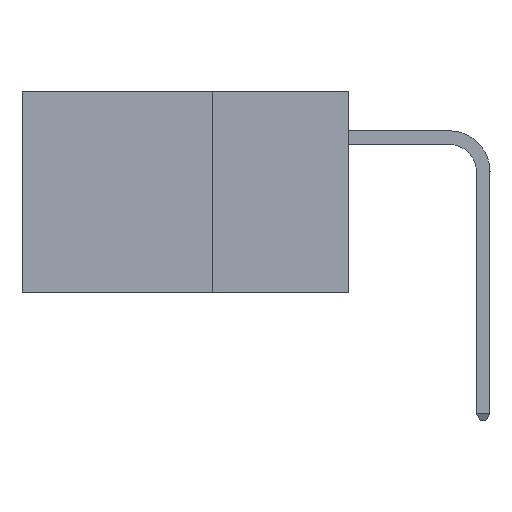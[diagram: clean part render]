
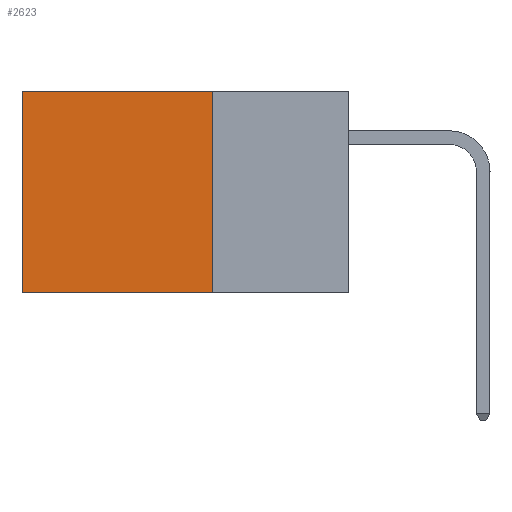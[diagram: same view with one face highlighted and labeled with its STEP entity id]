
A CAD part, left-side view. The second image highlights one B-rep face of the part: STEP entity #2623.
In plain terms, the highlighted planar face has unit normal (-1, 0, 0).
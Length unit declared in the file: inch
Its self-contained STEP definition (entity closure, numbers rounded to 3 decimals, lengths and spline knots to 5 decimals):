
#65 = PLANE ( 'NONE',  #16703 ) ;
#685 = EDGE_CURVE ( 'NONE', #5676, #15614, #16072, .T. ) ;
#888 = CARTESIAN_POINT ( 'NONE',  ( 0.2875, 0.25, -0.37 ) ) ;
#1685 = LINE ( 'NONE', #12060, #8061 ) ;
#2623 = ADVANCED_FACE ( 'NONE', ( #10730 ), #65, .F. ) ;
#2797 = CARTESIAN_POINT ( 'NONE',  ( 0.2875, 0.6, 0. ) ) ;
#3074 = EDGE_CURVE ( 'NONE', #14220, #5676, #1685, .T. ) ;
#3084 = VECTOR ( 'NONE', #14270, 39.37008 ) ;
#3350 = DIRECTION ( 'NONE',  ( 0., 0., -1. ) ) ;
#4287 = ORIENTED_EDGE ( 'NONE', *, *, #4540, .F. ) ;
#4376 = EDGE_CURVE ( 'NONE', #17453, #15614, #14077, .T. ) ;
#4540 = EDGE_CURVE ( 'NONE', #14220, #17453, #7182, .T. ) ;
#4625 = VECTOR ( 'NONE', #8269, 39.37008 ) ;
#4781 = DIRECTION ( 'NONE',  ( 0., 1., 0. ) ) ;
#5318 = ORIENTED_EDGE ( 'NONE', *, *, #3074, .T. ) ;
#5676 = VERTEX_POINT ( 'NONE', #7471 ) ;
#6261 = DIRECTION ( 'NONE',  ( 1., 0., 0. ) ) ;
#7182 = LINE ( 'NONE', #14359, #3084 ) ;
#7471 = CARTESIAN_POINT ( 'NONE',  ( 0.2875, 0.6, 0. ) ) ;
#8061 = VECTOR ( 'NONE', #4781, 39.37008 ) ;
#8269 = DIRECTION ( 'NONE',  ( 0., 1., 0. ) ) ;
#9499 = CARTESIAN_POINT ( 'NONE',  ( 0.2875, 0.25, 0. ) ) ;
#9553 = ORIENTED_EDGE ( 'NONE', *, *, #4376, .F. ) ;
#10077 = DIRECTION ( 'NONE',  ( 0., 0., -1. ) ) ;
#10730 = FACE_OUTER_BOUND ( 'NONE', #14315, .T. ) ;
#10827 = CARTESIAN_POINT ( 'NONE',  ( 0.2875, 0.25, -0.37 ) ) ;
#11514 = CARTESIAN_POINT ( 'NONE',  ( 0.2875, 0.6, -0.37 ) ) ;
#12060 = CARTESIAN_POINT ( 'NONE',  ( 0.2875, 0.25, 0. ) ) ;
#13913 = VECTOR ( 'NONE', #10077, 39.37008 ) ;
#14077 = LINE ( 'NONE', #888, #4625 ) ;
#14220 = VERTEX_POINT ( 'NONE', #9499 ) ;
#14270 = DIRECTION ( 'NONE',  ( 0., 0., -1. ) ) ;
#14315 = EDGE_LOOP ( 'NONE', ( #17378, #9553, #4287, #5318 ) ) ;
#14359 = CARTESIAN_POINT ( 'NONE',  ( 0.2875, 0.25, 0. ) ) ;
#15614 = VERTEX_POINT ( 'NONE', #11514 ) ;
#16072 = LINE ( 'NONE', #2797, #13913 ) ;
#16703 = AXIS2_PLACEMENT_3D ( 'NONE', #17980, #6261, #3350 ) ;
#17378 = ORIENTED_EDGE ( 'NONE', *, *, #685, .T. ) ;
#17453 = VERTEX_POINT ( 'NONE', #10827 ) ;
#17980 = CARTESIAN_POINT ( 'NONE',  ( 0.2875, 0.25, 0. ) ) ;
